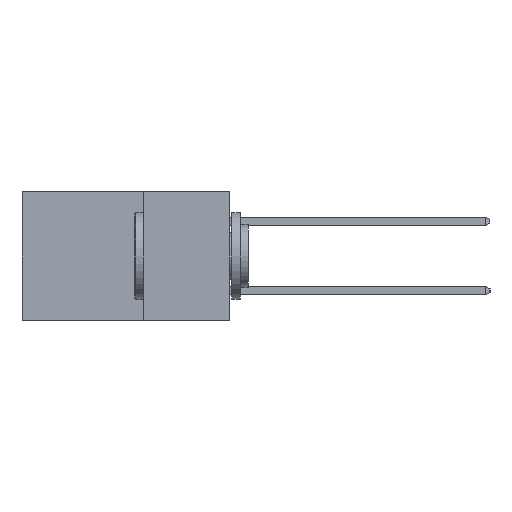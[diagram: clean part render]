
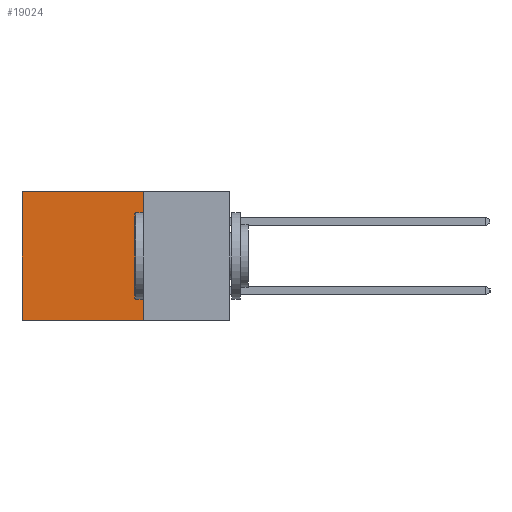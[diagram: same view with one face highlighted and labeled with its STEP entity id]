
A CAD part, left-side view. The second image highlights one B-rep face of the part: STEP entity #19024.
In plain terms, the highlighted planar face has unit normal (-1, 0, 0).
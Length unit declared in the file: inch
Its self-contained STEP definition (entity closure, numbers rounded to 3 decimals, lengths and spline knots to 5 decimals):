
#20 = CARTESIAN_POINT ( 'NONE',  ( 0.2615, 0.25, -0.37 ) ) ;
#1187 = LINE ( 'NONE', #9620, #17163 ) ;
#1391 = ORIENTED_EDGE ( 'NONE', *, *, #6590, .T. ) ;
#1966 = CARTESIAN_POINT ( 'NONE',  ( 0.2615, 0.25, -0.37 ) ) ;
#2051 = LINE ( 'NONE', #15165, #10257 ) ;
#3082 = CARTESIAN_POINT ( 'NONE',  ( 0.2615, 0.25, 0. ) ) ;
#3157 = DIRECTION ( 'NONE',  ( 0., 1., 0. ) ) ;
#3997 = ORIENTED_EDGE ( 'NONE', *, *, #10779, .T. ) ;
#5907 = VERTEX_POINT ( 'NONE', #12229 ) ;
#6445 = DIRECTION ( 'NONE',  ( 1., 0., 0. ) ) ;
#6590 = EDGE_CURVE ( 'NONE', #17938, #6846, #2051, .T. ) ;
#6846 = VERTEX_POINT ( 'NONE', #9889 ) ;
#7373 = EDGE_LOOP ( 'NONE', ( #1391, #14290, #12371, #3997 ) ) ;
#7539 = AXIS2_PLACEMENT_3D ( 'NONE', #10994, #6445, #17199 ) ;
#7624 = VECTOR ( 'NONE', #3157, 39.37008 ) ;
#9272 = FACE_OUTER_BOUND ( 'NONE', #7373, .T. ) ;
#9620 = CARTESIAN_POINT ( 'NONE',  ( 0.2615, 0.25, -0.37 ) ) ;
#9889 = CARTESIAN_POINT ( 'NONE',  ( 0.2615, 0.6, -0.37 ) ) ;
#10005 = CARTESIAN_POINT ( 'NONE',  ( 0.2615, 0.6, 0. ) ) ;
#10038 = VECTOR ( 'NONE', #14334, 39.37008 ) ;
#10257 = VECTOR ( 'NONE', #16708, 39.37008 ) ;
#10521 = LINE ( 'NONE', #1966, #10038 ) ;
#10779 = EDGE_CURVE ( 'NONE', #5907, #17938, #15828, .T. ) ;
#10821 = VERTEX_POINT ( 'NONE', #20 ) ;
#10994 = CARTESIAN_POINT ( 'NONE',  ( 0.2615, 0.25, -0.37 ) ) ;
#12229 = CARTESIAN_POINT ( 'NONE',  ( 0.2615, 0.25, 0. ) ) ;
#12371 = ORIENTED_EDGE ( 'NONE', *, *, #14107, .F. ) ;
#14107 = EDGE_CURVE ( 'NONE', #5907, #10821, #1187, .T. ) ;
#14290 = ORIENTED_EDGE ( 'NONE', *, *, #18396, .F. ) ;
#14334 = DIRECTION ( 'NONE',  ( 0., 1., 0. ) ) ;
#14364 = DIRECTION ( 'NONE',  ( 0., 0., -1. ) ) ;
#15165 = CARTESIAN_POINT ( 'NONE',  ( 0.2615, 0.6, -0.37 ) ) ;
#15655 = PLANE ( 'NONE',  #7539 ) ;
#15828 = LINE ( 'NONE', #3082, #7624 ) ;
#16708 = DIRECTION ( 'NONE',  ( 0., 0., -1. ) ) ;
#17163 = VECTOR ( 'NONE', #14364, 39.37008 ) ;
#17199 = DIRECTION ( 'NONE',  ( 0., 0., -1. ) ) ;
#17938 = VERTEX_POINT ( 'NONE', #10005 ) ;
#18396 = EDGE_CURVE ( 'NONE', #10821, #6846, #10521, .T. ) ;
#19024 = ADVANCED_FACE ( 'NONE', ( #9272 ), #15655, .F. ) ;
